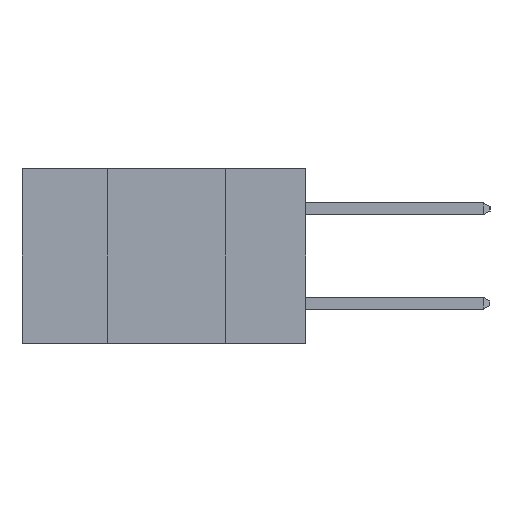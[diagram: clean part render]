
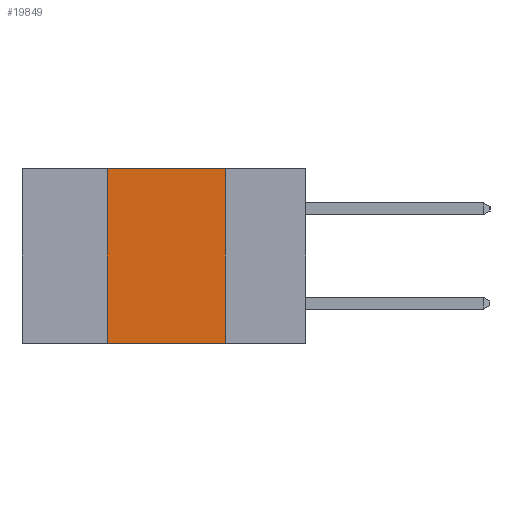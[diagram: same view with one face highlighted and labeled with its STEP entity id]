
A CAD part, left-side view. The second image highlights one B-rep face of the part: STEP entity #19849.
In plain terms, the highlighted planar face has unit normal (-1, 0, 0).
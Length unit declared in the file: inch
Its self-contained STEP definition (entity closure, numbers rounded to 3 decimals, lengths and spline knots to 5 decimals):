
#86 = CARTESIAN_POINT ( 'NONE',  ( 0., 0.42, 0. ) ) ;
#833 = ORIENTED_EDGE ( 'NONE', *, *, #12860, .F. ) ;
#1100 = ORIENTED_EDGE ( 'NONE', *, *, #13956, .F. ) ;
#1155 = CARTESIAN_POINT ( 'NONE',  ( 0., 0.42, -0.37 ) ) ;
#1180 = VERTEX_POINT ( 'NONE', #14325 ) ;
#1186 = LINE ( 'NONE', #86, #5094 ) ;
#1632 = DIRECTION ( 'NONE',  ( 0., -1., 0. ) ) ;
#3139 = LINE ( 'NONE', #9862, #11386 ) ;
#3321 = EDGE_LOOP ( 'NONE', ( #1100, #18448, #833, #16163 ) ) ;
#4339 = AXIS2_PLACEMENT_3D ( 'NONE', #7887, #19151, #9524 ) ;
#4878 = VECTOR ( 'NONE', #6485, 39.37008 ) ;
#5094 = VECTOR ( 'NONE', #5147, 39.37008 ) ;
#5147 = DIRECTION ( 'NONE',  ( 0., 0., 1. ) ) ;
#6485 = DIRECTION ( 'NONE',  ( 0., -1., 0. ) ) ;
#6581 = CARTESIAN_POINT ( 'NONE',  ( 0., 0.17, 0. ) ) ;
#7163 = CARTESIAN_POINT ( 'NONE',  ( 0., 0.17, -0.37 ) ) ;
#7887 = CARTESIAN_POINT ( 'NONE',  ( 0., 0.6, 0. ) ) ;
#9175 = VECTOR ( 'NONE', #21044, 39.37008 ) ;
#9524 = DIRECTION ( 'NONE',  ( 0., 0., -1. ) ) ;
#9862 = CARTESIAN_POINT ( 'NONE',  ( 0., 0.6, 0. ) ) ;
#11376 = VERTEX_POINT ( 'NONE', #18355 ) ;
#11386 = VECTOR ( 'NONE', #1632, 39.37008 ) ;
#11805 = EDGE_CURVE ( 'NONE', #14426, #13665, #16809, .T. ) ;
#12860 = EDGE_CURVE ( 'NONE', #14426, #11376, #1186, .T. ) ;
#13464 = LINE ( 'NONE', #6581, #9175 ) ;
#13665 = VERTEX_POINT ( 'NONE', #7163 ) ;
#13956 = EDGE_CURVE ( 'NONE', #1180, #13665, #13464, .T. ) ;
#14325 = CARTESIAN_POINT ( 'NONE',  ( 0., 0.17, 0. ) ) ;
#14426 = VERTEX_POINT ( 'NONE', #1155 ) ;
#16163 = ORIENTED_EDGE ( 'NONE', *, *, #11805, .T. ) ;
#16809 = LINE ( 'NONE', #20892, #4878 ) ;
#17524 = PLANE ( 'NONE',  #4339 ) ;
#18035 = EDGE_CURVE ( 'NONE', #11376, #1180, #3139, .T. ) ;
#18355 = CARTESIAN_POINT ( 'NONE',  ( 0., 0.42, 0. ) ) ;
#18448 = ORIENTED_EDGE ( 'NONE', *, *, #18035, .F. ) ;
#19151 = DIRECTION ( 'NONE',  ( 1., 0., 0. ) ) ;
#19849 = ADVANCED_FACE ( 'NONE', ( #20095 ), #17524, .F. ) ;
#20095 = FACE_OUTER_BOUND ( 'NONE', #3321, .T. ) ;
#20892 = CARTESIAN_POINT ( 'NONE',  ( 0., 0.6, -0.37 ) ) ;
#21044 = DIRECTION ( 'NONE',  ( 0., 0., -1. ) ) ;
